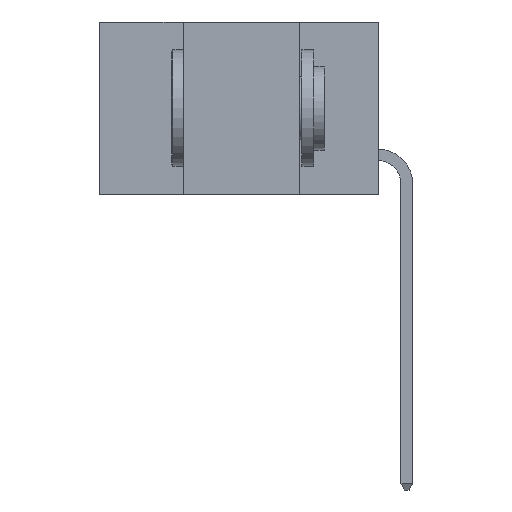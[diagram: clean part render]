
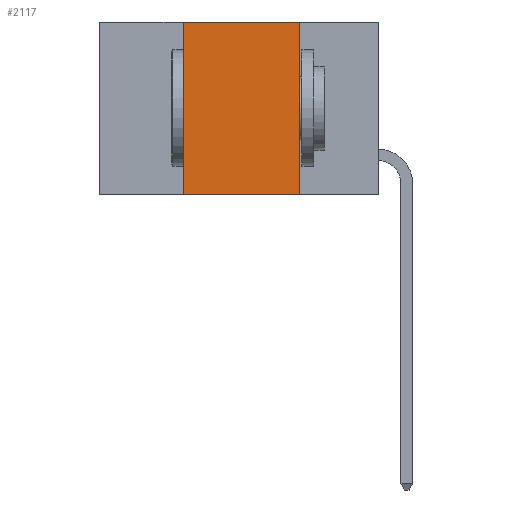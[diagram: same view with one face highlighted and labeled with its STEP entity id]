
A CAD part, left-side view. The second image highlights one B-rep face of the part: STEP entity #2117.
In plain terms, the highlighted planar face has unit normal (-1, 0, 0).
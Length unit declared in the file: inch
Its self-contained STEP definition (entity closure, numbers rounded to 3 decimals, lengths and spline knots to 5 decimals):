
#641 = FACE_OUTER_BOUND ( 'NONE', #4666, .T. ) ;
#747 = AXIS2_PLACEMENT_3D ( 'NONE', #6180, #12554, #9430 ) ;
#887 = CARTESIAN_POINT ( 'NONE',  ( 0., 0.6, 0. ) ) ;
#2034 = VECTOR ( 'NONE', #2075, 39.37008 ) ;
#2073 = VECTOR ( 'NONE', #15132, 39.37008 ) ;
#2075 = DIRECTION ( 'NONE',  ( 0., -1., 0. ) ) ;
#2117 = ADVANCED_FACE ( 'NONE', ( #641 ), #6822, .F. ) ;
#2407 = CARTESIAN_POINT ( 'NONE',  ( 0., 0.42, -0.37 ) ) ;
#3118 = CARTESIAN_POINT ( 'NONE',  ( 0., 0.42, 0. ) ) ;
#3247 = EDGE_CURVE ( 'NONE', #11753, #5193, #7856, .T. ) ;
#3751 = LINE ( 'NONE', #8950, #6677 ) ;
#3987 = ORIENTED_EDGE ( 'NONE', *, *, #14968, .F. ) ;
#4249 = CARTESIAN_POINT ( 'NONE',  ( 0., 0.17, 0. ) ) ;
#4250 = EDGE_CURVE ( 'NONE', #11624, #5193, #3751, .T. ) ;
#4666 = EDGE_LOOP ( 'NONE', ( #6543, #3987, #7685, #11597 ) ) ;
#4875 = LINE ( 'NONE', #887, #2034 ) ;
#5033 = CARTESIAN_POINT ( 'NONE',  ( 0., 0.17, -0.37 ) ) ;
#5193 = VERTEX_POINT ( 'NONE', #5033 ) ;
#6107 = LINE ( 'NONE', #2407, #11739 ) ;
#6180 = CARTESIAN_POINT ( 'NONE',  ( 0., 0.6, 0. ) ) ;
#6543 = ORIENTED_EDGE ( 'NONE', *, *, #4250, .F. ) ;
#6677 = VECTOR ( 'NONE', #8945, 39.37008 ) ;
#6822 = PLANE ( 'NONE',  #747 ) ;
#7005 = CARTESIAN_POINT ( 'NONE',  ( 0., 0.42, -0.37 ) ) ;
#7685 = ORIENTED_EDGE ( 'NONE', *, *, #14470, .F. ) ;
#7856 = LINE ( 'NONE', #15283, #2073 ) ;
#8945 = DIRECTION ( 'NONE',  ( 0., 0., -1. ) ) ;
#8950 = CARTESIAN_POINT ( 'NONE',  ( 0., 0.17, -0.37 ) ) ;
#9430 = DIRECTION ( 'NONE',  ( 0., 0., -1. ) ) ;
#9743 = DIRECTION ( 'NONE',  ( 0., 0., 1. ) ) ;
#11032 = VERTEX_POINT ( 'NONE', #3118 ) ;
#11597 = ORIENTED_EDGE ( 'NONE', *, *, #3247, .T. ) ;
#11624 = VERTEX_POINT ( 'NONE', #4249 ) ;
#11739 = VECTOR ( 'NONE', #9743, 39.37008 ) ;
#11753 = VERTEX_POINT ( 'NONE', #7005 ) ;
#12554 = DIRECTION ( 'NONE',  ( 1., 0., 0. ) ) ;
#14470 = EDGE_CURVE ( 'NONE', #11753, #11032, #6107, .T. ) ;
#14968 = EDGE_CURVE ( 'NONE', #11032, #11624, #4875, .T. ) ;
#15132 = DIRECTION ( 'NONE',  ( 0., -1., 0. ) ) ;
#15283 = CARTESIAN_POINT ( 'NONE',  ( 0., 0.6, -0.37 ) ) ;
